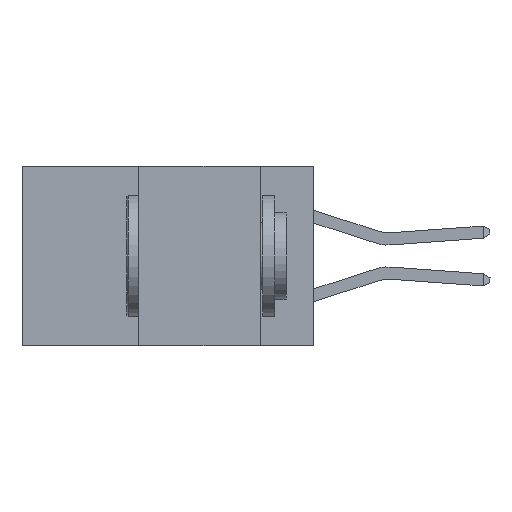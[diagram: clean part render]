
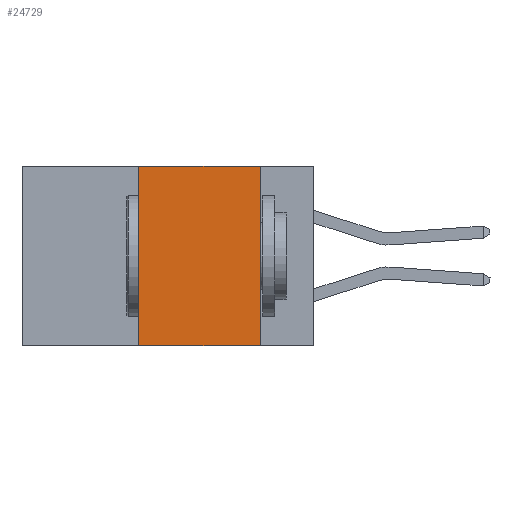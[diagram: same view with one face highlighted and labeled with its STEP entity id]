
A CAD part, left-side view. The second image highlights one B-rep face of the part: STEP entity #24729.
In plain terms, the highlighted planar face has unit normal (-1, 0, 0).
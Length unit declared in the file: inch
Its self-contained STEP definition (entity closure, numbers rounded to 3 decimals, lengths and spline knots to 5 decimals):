
#563 = CARTESIAN_POINT ( 'NONE',  ( 0., 0.11, 0. ) ) ;
#614 = EDGE_CURVE ( 'NONE', #4458, #22289, #11452, .T. ) ;
#675 = EDGE_LOOP ( 'NONE', ( #25726, #11566, #24086, #22043 ) ) ;
#934 = VECTOR ( 'NONE', #9075, 39.37008 ) ;
#963 = VECTOR ( 'NONE', #10001, 39.37008 ) ;
#1350 = CARTESIAN_POINT ( 'NONE',  ( 0., 0.36, -0.37 ) ) ;
#2946 = LINE ( 'NONE', #3136, #23018 ) ;
#3136 = CARTESIAN_POINT ( 'NONE',  ( 0., 0.6, 0. ) ) ;
#3235 = VERTEX_POINT ( 'NONE', #24385 ) ;
#3334 = EDGE_CURVE ( 'NONE', #22215, #3235, #9416, .T. ) ;
#4142 = CARTESIAN_POINT ( 'NONE',  ( 0., 0.36, 0. ) ) ;
#4458 = VERTEX_POINT ( 'NONE', #563 ) ;
#4575 = VECTOR ( 'NONE', #23965, 39.37008 ) ;
#5202 = CARTESIAN_POINT ( 'NONE',  ( 0., 0.11, -0.37 ) ) ;
#5609 = FACE_OUTER_BOUND ( 'NONE', #675, .T. ) ;
#6917 = DIRECTION ( 'NONE',  ( 0., -1., 0. ) ) ;
#9075 = DIRECTION ( 'NONE',  ( 0., -1., 0. ) ) ;
#9416 = LINE ( 'NONE', #4142, #963 ) ;
#10001 = DIRECTION ( 'NONE',  ( 0., 0., 1. ) ) ;
#11452 = LINE ( 'NONE', #15897, #4575 ) ;
#11566 = ORIENTED_EDGE ( 'NONE', *, *, #13736, .F. ) ;
#11923 = PLANE ( 'NONE',  #24494 ) ;
#12277 = DIRECTION ( 'NONE',  ( 1., 0., 0. ) ) ;
#13736 = EDGE_CURVE ( 'NONE', #3235, #4458, #2946, .T. ) ;
#15897 = CARTESIAN_POINT ( 'NONE',  ( 0., 0.11, 0. ) ) ;
#16010 = DIRECTION ( 'NONE',  ( 0., 0., -1. ) ) ;
#18305 = CARTESIAN_POINT ( 'NONE',  ( 0., 0.6, 0. ) ) ;
#21132 = CARTESIAN_POINT ( 'NONE',  ( 0., 0.6, -0.37 ) ) ;
#21353 = LINE ( 'NONE', #21132, #934 ) ;
#22043 = ORIENTED_EDGE ( 'NONE', *, *, #26042, .T. ) ;
#22215 = VERTEX_POINT ( 'NONE', #1350 ) ;
#22289 = VERTEX_POINT ( 'NONE', #5202 ) ;
#23018 = VECTOR ( 'NONE', #6917, 39.37008 ) ;
#23965 = DIRECTION ( 'NONE',  ( 0., 0., -1. ) ) ;
#24086 = ORIENTED_EDGE ( 'NONE', *, *, #3334, .F. ) ;
#24385 = CARTESIAN_POINT ( 'NONE',  ( 0., 0.36, 0. ) ) ;
#24494 = AXIS2_PLACEMENT_3D ( 'NONE', #18305, #12277, #16010 ) ;
#24729 = ADVANCED_FACE ( 'NONE', ( #5609 ), #11923, .F. ) ;
#25726 = ORIENTED_EDGE ( 'NONE', *, *, #614, .F. ) ;
#26042 = EDGE_CURVE ( 'NONE', #22215, #22289, #21353, .T. ) ;
